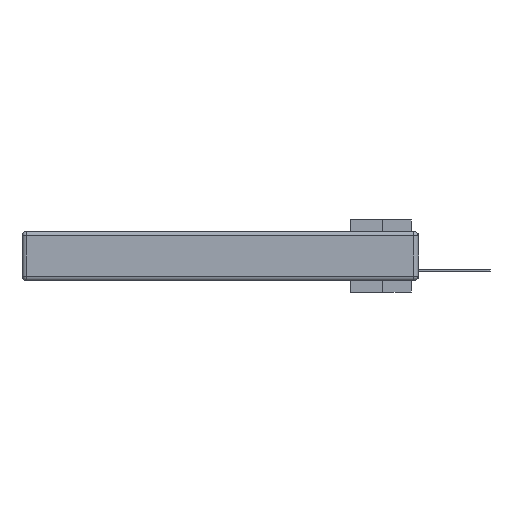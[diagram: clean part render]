
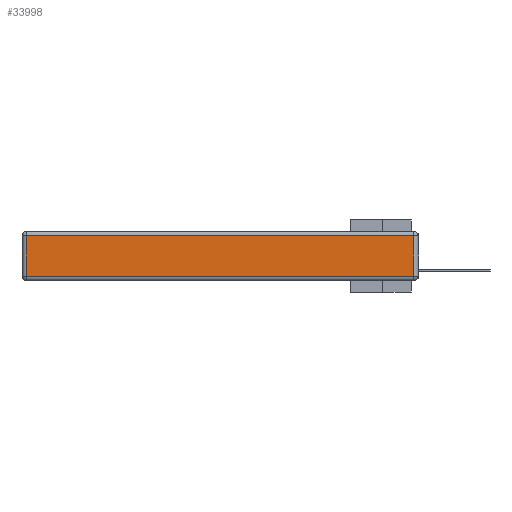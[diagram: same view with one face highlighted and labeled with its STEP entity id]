
A CAD part, left-side view. The second image highlights one B-rep face of the part: STEP entity #33998.
In plain terms, the highlighted planar face has unit normal (-1, 0, 0).
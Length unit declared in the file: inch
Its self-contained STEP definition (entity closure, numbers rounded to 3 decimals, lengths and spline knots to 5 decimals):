
#1719 = AXIS2_PLACEMENT_3D ( 'NONE', #29173, #26577, #21372 ) ;
#1725 = CARTESIAN_POINT ( 'NONE',  ( 0., 0.03, -0.313 ) ) ;
#2230 = CARTESIAN_POINT ( 'NONE',  ( 0., 2.72, -0.343 ) ) ;
#2967 = DIRECTION ( 'NONE',  ( 0., -1., 0. ) ) ;
#3128 = CARTESIAN_POINT ( 'NONE',  ( 0., 0., -0.313 ) ) ;
#3764 = CARTESIAN_POINT ( 'NONE',  ( 0., 2.72, -0.313 ) ) ;
#3886 = EDGE_LOOP ( 'NONE', ( #16891, #31548, #27298, #10604 ) ) ;
#4060 = VECTOR ( 'NONE', #2967, 39.37008 ) ;
#5567 = LINE ( 'NONE', #3128, #4060 ) ;
#6345 = EDGE_CURVE ( 'NONE', #21776, #19896, #15533, .T. ) ;
#8234 = DIRECTION ( 'NONE',  ( 0., 0., 1. ) ) ;
#8249 = EDGE_CURVE ( 'NONE', #23613, #10502, #5567, .T. ) ;
#9843 = CARTESIAN_POINT ( 'NONE',  ( 0., 2.72, -0.03 ) ) ;
#10502 = VERTEX_POINT ( 'NONE', #1725 ) ;
#10604 = ORIENTED_EDGE ( 'NONE', *, *, #21123, .T. ) ;
#11191 = CARTESIAN_POINT ( 'NONE',  ( 0., 0.03, -0.343 ) ) ;
#15174 = VECTOR ( 'NONE', #28555, 39.37008 ) ;
#15533 = LINE ( 'NONE', #31524, #15174 ) ;
#16891 = ORIENTED_EDGE ( 'NONE', *, *, #8249, .T. ) ;
#17111 = VECTOR ( 'NONE', #8234, 39.37008 ) ;
#18587 = PLANE ( 'NONE',  #1719 ) ;
#19896 = VERTEX_POINT ( 'NONE', #9843 ) ;
#21123 = EDGE_CURVE ( 'NONE', #19896, #23613, #32331, .T. ) ;
#21134 = LINE ( 'NONE', #11191, #17111 ) ;
#21313 = CARTESIAN_POINT ( 'NONE',  ( 0., 0.03, -0.03 ) ) ;
#21372 = DIRECTION ( 'NONE',  ( 0., 0., 1. ) ) ;
#21776 = VERTEX_POINT ( 'NONE', #21313 ) ;
#22581 = EDGE_CURVE ( 'NONE', #10502, #21776, #21134, .T. ) ;
#23613 = VERTEX_POINT ( 'NONE', #3764 ) ;
#24264 = VECTOR ( 'NONE', #26230, 39.37008 ) ;
#26230 = DIRECTION ( 'NONE',  ( 0., 0., -1. ) ) ;
#26577 = DIRECTION ( 'NONE',  ( -1., 0., 0. ) ) ;
#27298 = ORIENTED_EDGE ( 'NONE', *, *, #6345, .T. ) ;
#28555 = DIRECTION ( 'NONE',  ( 0., 1., 0. ) ) ;
#29173 = CARTESIAN_POINT ( 'NONE',  ( 0., 0., -0.343 ) ) ;
#31524 = CARTESIAN_POINT ( 'NONE',  ( 0., 2.75, -0.03 ) ) ;
#31548 = ORIENTED_EDGE ( 'NONE', *, *, #22581, .T. ) ;
#31809 = FACE_OUTER_BOUND ( 'NONE', #3886, .T. ) ;
#32331 = LINE ( 'NONE', #2230, #24264 ) ;
#33998 = ADVANCED_FACE ( 'NONE', ( #31809 ), #18587, .T. ) ;
